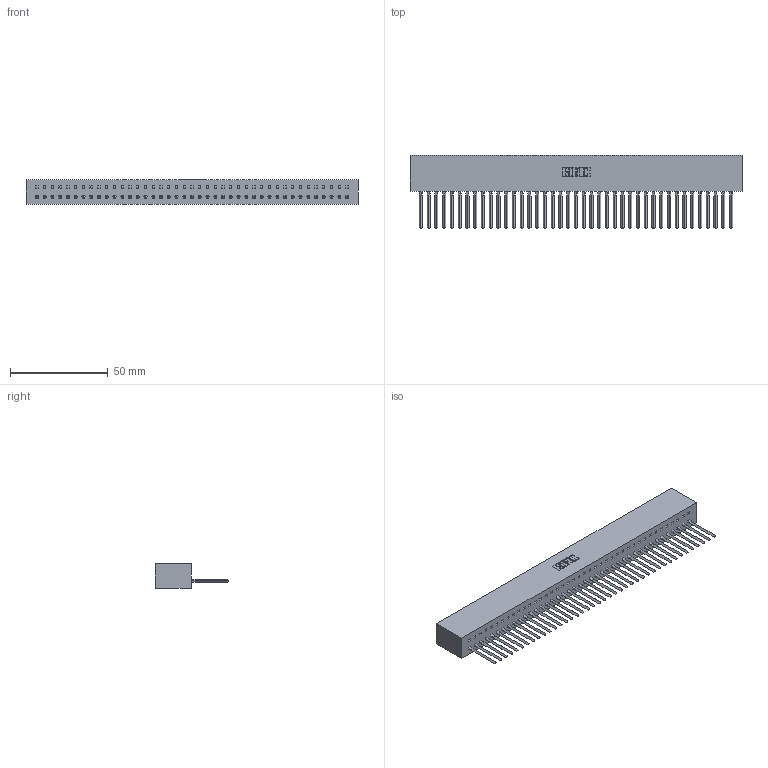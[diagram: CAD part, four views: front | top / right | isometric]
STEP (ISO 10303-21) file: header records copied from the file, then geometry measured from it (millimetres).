
FILE_DESCRIPTION (( 'STEP AP203' ), '1' );
FILE_NAME ('317-041-541-601.STEP', '2020-02-28T00:54:05', ( '' ), ( '' ), 'SwSTEP 2.0', 'SolidWorks 2016', '' );
FILE_SCHEMA (( 'CONFIG_CONTROL_DESIGN' ));
Length unit declared in the file: inch
Products named in the file (3): 317-041-541-601; 317 Part_Lugless; 317-290-002_541
Assembly tree (42 placements, depth 2):
  317-041-541-601
    317 Part_Lugless
    317-290-002_541  x41
Bounding box: 169.67 x 37.34 x 12.7 mm (x, y, z)
Volume: 29190.2 mm3; surface area: 41408 mm2
Topology: 42 solids, 42 shells, 6322 faces, 18033 edges, 11720 vertices
Faces by surface type: plane 5134, cylinder 1024, bspline 164
Entity records: 59232 total; most frequent: CARTESIAN_POINT 11172, ORIENTED_EDGE 10466, DIRECTION 8587, EDGE_CURVE 5233, LINE 4877, VECTOR 4877, VERTEX_POINT 3480, AXIS2_PLACEMENT_3D 1855
